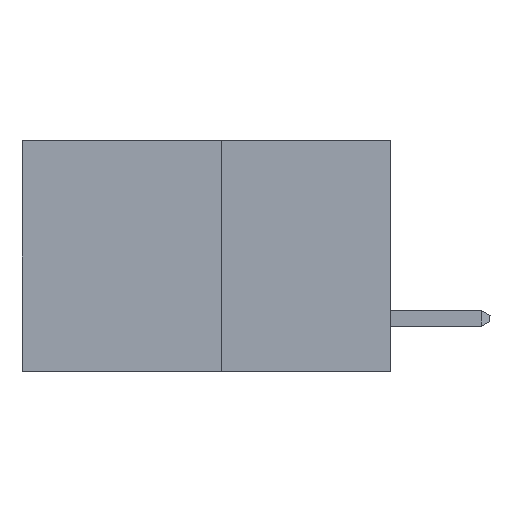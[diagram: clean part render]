
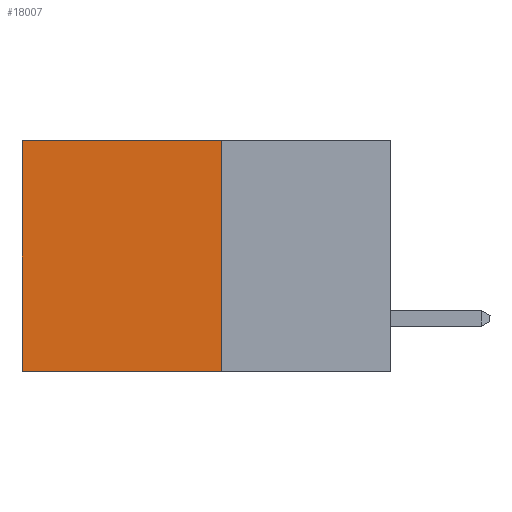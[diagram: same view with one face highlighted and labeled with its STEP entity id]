
A CAD part, left-side view. The second image highlights one B-rep face of the part: STEP entity #18007.
In plain terms, the highlighted planar face has unit normal (-1, 0, 0).
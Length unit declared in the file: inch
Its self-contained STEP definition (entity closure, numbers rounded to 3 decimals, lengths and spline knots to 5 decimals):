
#250 = CARTESIAN_POINT ( 'NONE',  ( 0.277, 0.27, -0.37 ) ) ;
#990 = VECTOR ( 'NONE', #12859, 39.37008 ) ;
#1836 = CARTESIAN_POINT ( 'NONE',  ( 0.277, 0.59, -0.37 ) ) ;
#2356 = ORIENTED_EDGE ( 'NONE', *, *, #25720, .T. ) ;
#2450 = LINE ( 'NONE', #13229, #18442 ) ;
#3118 = PLANE ( 'NONE',  #5058 ) ;
#3421 = EDGE_CURVE ( 'NONE', #24249, #9348, #25248, .T. ) ;
#4923 = ORIENTED_EDGE ( 'NONE', *, *, #3421, .T. ) ;
#5058 = AXIS2_PLACEMENT_3D ( 'NONE', #23714, #17701, #5256 ) ;
#5065 = ORIENTED_EDGE ( 'NONE', *, *, #12091, .F. ) ;
#5256 = DIRECTION ( 'NONE',  ( 0., 0., -1. ) ) ;
#6122 = VERTEX_POINT ( 'NONE', #22032 ) ;
#7769 = LINE ( 'NONE', #250, #23501 ) ;
#9348 = VERTEX_POINT ( 'NONE', #1836 ) ;
#10085 = CARTESIAN_POINT ( 'NONE',  ( 0.277, 0.27, -0.37 ) ) ;
#10276 = ORIENTED_EDGE ( 'NONE', *, *, #15186, .F. ) ;
#10853 = DIRECTION ( 'NONE',  ( 0., 1., 0. ) ) ;
#12091 = EDGE_CURVE ( 'NONE', #6122, #18901, #17648, .T. ) ;
#12859 = DIRECTION ( 'NONE',  ( 0., 0., -1. ) ) ;
#13229 = CARTESIAN_POINT ( 'NONE',  ( 0.277, 0.27, 0. ) ) ;
#15186 = EDGE_CURVE ( 'NONE', #18901, #9348, #7769, .T. ) ;
#15325 = DIRECTION ( 'NONE',  ( 0., 1., 0. ) ) ;
#16926 = CARTESIAN_POINT ( 'NONE',  ( 0.277, 0.27, -0.37 ) ) ;
#17129 = EDGE_LOOP ( 'NONE', ( #4923, #10276, #5065, #2356 ) ) ;
#17648 = LINE ( 'NONE', #16926, #990 ) ;
#17701 = DIRECTION ( 'NONE',  ( 1., 0., 0. ) ) ;
#18007 = ADVANCED_FACE ( 'NONE', ( #24487 ), #3118, .F. ) ;
#18442 = VECTOR ( 'NONE', #15325, 39.37008 ) ;
#18901 = VERTEX_POINT ( 'NONE', #10085 ) ;
#19267 = VECTOR ( 'NONE', #23946, 39.37008 ) ;
#22032 = CARTESIAN_POINT ( 'NONE',  ( 0.277, 0.27, 0. ) ) ;
#23501 = VECTOR ( 'NONE', #10853, 39.37008 ) ;
#23714 = CARTESIAN_POINT ( 'NONE',  ( 0.277, 0.27, -0.37 ) ) ;
#23946 = DIRECTION ( 'NONE',  ( 0., 0., -1. ) ) ;
#24249 = VERTEX_POINT ( 'NONE', #24825 ) ;
#24487 = FACE_OUTER_BOUND ( 'NONE', #17129, .T. ) ;
#24825 = CARTESIAN_POINT ( 'NONE',  ( 0.277, 0.59, 0. ) ) ;
#25059 = CARTESIAN_POINT ( 'NONE',  ( 0.277, 0.59, -0.37 ) ) ;
#25248 = LINE ( 'NONE', #25059, #19267 ) ;
#25720 = EDGE_CURVE ( 'NONE', #6122, #24249, #2450, .T. ) ;
